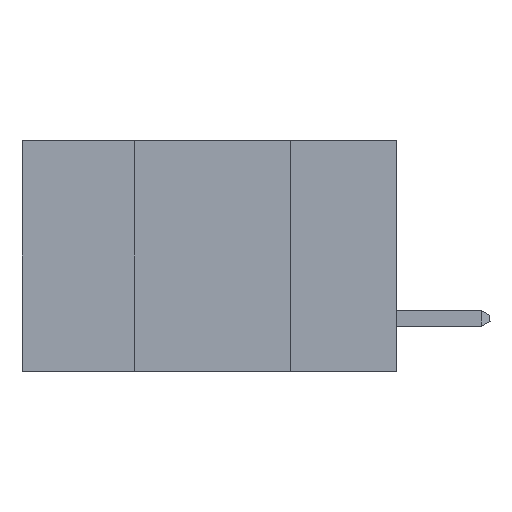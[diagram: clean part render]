
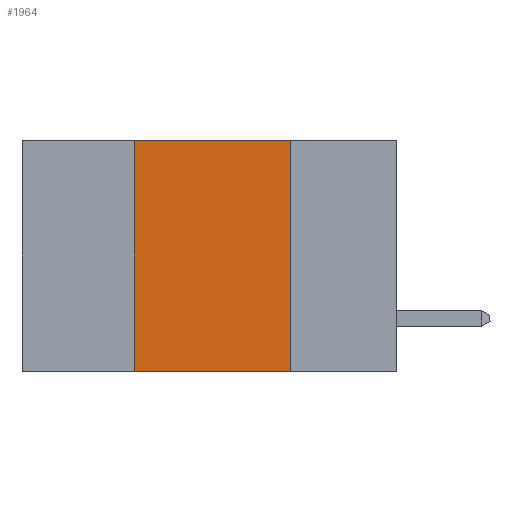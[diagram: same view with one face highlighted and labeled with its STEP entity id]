
A CAD part, left-side view. The second image highlights one B-rep face of the part: STEP entity #1964.
In plain terms, the highlighted planar face has unit normal (-1, 0, 0).
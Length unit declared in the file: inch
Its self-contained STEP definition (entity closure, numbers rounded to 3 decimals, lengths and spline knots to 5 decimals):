
#51 = CARTESIAN_POINT ( 'NONE',  ( 0., 0.17, 0. ) ) ;
#310 = VERTEX_POINT ( 'NONE', #13114 ) ;
#449 = DIRECTION ( 'NONE',  ( 1., 0., 0. ) ) ;
#1345 = CARTESIAN_POINT ( 'NONE',  ( 0., 0.42, -0.37 ) ) ;
#1758 = EDGE_CURVE ( 'NONE', #10395, #310, #12048, .T. ) ;
#1964 = ADVANCED_FACE ( 'NONE', ( #6864 ), #9191, .F. ) ;
#2933 = EDGE_CURVE ( 'NONE', #310, #3325, #14748, .T. ) ;
#2953 = ORIENTED_EDGE ( 'NONE', *, *, #1758, .F. ) ;
#3325 = VERTEX_POINT ( 'NONE', #4136 ) ;
#4135 = DIRECTION ( 'NONE',  ( 0., 0., -1. ) ) ;
#4136 = CARTESIAN_POINT ( 'NONE',  ( 0., 0.17, 0. ) ) ;
#5674 = ORIENTED_EDGE ( 'NONE', *, *, #2933, .F. ) ;
#6045 = LINE ( 'NONE', #51, #14343 ) ;
#6111 = VECTOR ( 'NONE', #12562, 39.37008 ) ;
#6864 = FACE_OUTER_BOUND ( 'NONE', #8101, .T. ) ;
#7105 = VERTEX_POINT ( 'NONE', #7221 ) ;
#7221 = CARTESIAN_POINT ( 'NONE',  ( 0., 0.17, -0.37 ) ) ;
#8101 = EDGE_LOOP ( 'NONE', ( #14319, #5674, #2953, #12798 ) ) ;
#8162 = DIRECTION ( 'NONE',  ( 0., 0., 1. ) ) ;
#8711 = CARTESIAN_POINT ( 'NONE',  ( 0., 0.6, 0. ) ) ;
#9042 = VECTOR ( 'NONE', #8162, 39.37008 ) ;
#9191 = PLANE ( 'NONE',  #10825 ) ;
#9835 = EDGE_CURVE ( 'NONE', #10395, #7105, #14423, .T. ) ;
#10395 = VERTEX_POINT ( 'NONE', #1345 ) ;
#10734 = CARTESIAN_POINT ( 'NONE',  ( 0., 0.6, -0.37 ) ) ;
#10825 = AXIS2_PLACEMENT_3D ( 'NONE', #13925, #449, #4135 ) ;
#11169 = VECTOR ( 'NONE', #12965, 39.37008 ) ;
#11596 = CARTESIAN_POINT ( 'NONE',  ( 0., 0.42, 0. ) ) ;
#12048 = LINE ( 'NONE', #11596, #9042 ) ;
#12562 = DIRECTION ( 'NONE',  ( 0., -1., 0. ) ) ;
#12718 = DIRECTION ( 'NONE',  ( 0., 0., -1. ) ) ;
#12798 = ORIENTED_EDGE ( 'NONE', *, *, #9835, .T. ) ;
#12965 = DIRECTION ( 'NONE',  ( 0., -1., 0. ) ) ;
#13114 = CARTESIAN_POINT ( 'NONE',  ( 0., 0.42, 0. ) ) ;
#13284 = EDGE_CURVE ( 'NONE', #3325, #7105, #6045, .T. ) ;
#13925 = CARTESIAN_POINT ( 'NONE',  ( 0., 0.6, 0. ) ) ;
#14319 = ORIENTED_EDGE ( 'NONE', *, *, #13284, .F. ) ;
#14343 = VECTOR ( 'NONE', #12718, 39.37008 ) ;
#14423 = LINE ( 'NONE', #10734, #11169 ) ;
#14748 = LINE ( 'NONE', #8711, #6111 ) ;
